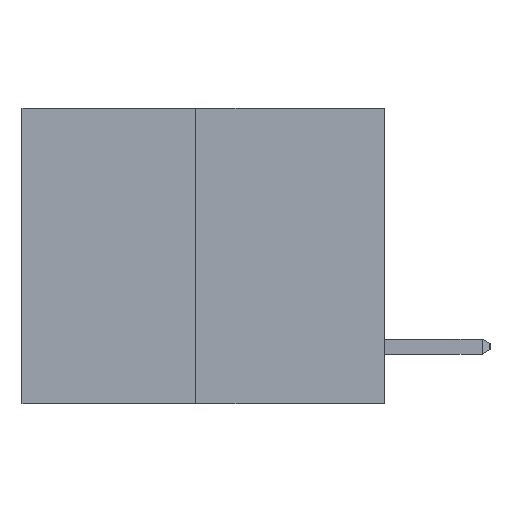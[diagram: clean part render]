
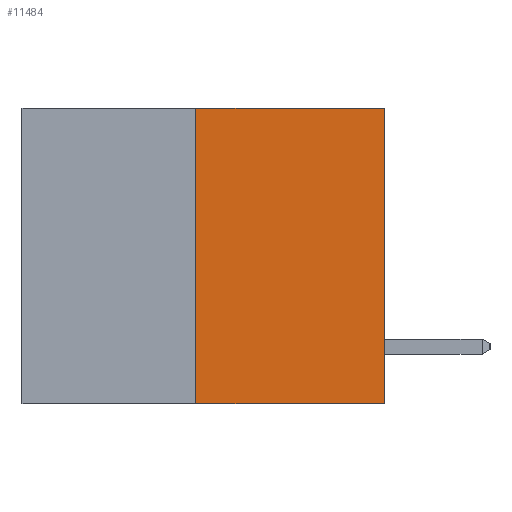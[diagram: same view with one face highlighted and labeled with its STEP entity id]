
A CAD part, left-side view. The second image highlights one B-rep face of the part: STEP entity #11484.
In plain terms, the highlighted planar face has unit normal (-1, 0, 0).
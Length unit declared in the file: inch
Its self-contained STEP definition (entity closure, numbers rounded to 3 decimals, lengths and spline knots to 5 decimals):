
#1360 = ORIENTED_EDGE ( 'NONE', *, *, #4857, .T. ) ;
#1458 = DIRECTION ( 'NONE',  ( 0., 0., 1. ) ) ;
#2323 = ORIENTED_EDGE ( 'NONE', *, *, #9073, .T. ) ;
#2783 = CARTESIAN_POINT ( 'NONE',  ( 0., 0.312, -0.49 ) ) ;
#3047 = VERTEX_POINT ( 'NONE', #7155 ) ;
#3718 = DIRECTION ( 'NONE',  ( 1., 0., 0. ) ) ;
#4088 = CARTESIAN_POINT ( 'NONE',  ( 0., 0., 0. ) ) ;
#4324 = CARTESIAN_POINT ( 'NONE',  ( 0., 0.312, 0. ) ) ;
#4562 = ORIENTED_EDGE ( 'NONE', *, *, #13847, .F. ) ;
#4671 = LINE ( 'NONE', #8353, #8855 ) ;
#4857 = EDGE_CURVE ( 'NONE', #11844, #3047, #4671, .T. ) ;
#4933 = DIRECTION ( 'NONE',  ( 0., 0., -1. ) ) ;
#5059 = CARTESIAN_POINT ( 'NONE',  ( 0., 0., 0. ) ) ;
#5150 = FACE_OUTER_BOUND ( 'NONE', #14146, .T. ) ;
#6136 = CARTESIAN_POINT ( 'NONE',  ( 0., 0.6, 0. ) ) ;
#6342 = DIRECTION ( 'NONE',  ( 0., 0., 1. ) ) ;
#7155 = CARTESIAN_POINT ( 'NONE',  ( 0., 0., -0.49 ) ) ;
#7371 = LINE ( 'NONE', #2783, #8485 ) ;
#8047 = CARTESIAN_POINT ( 'NONE',  ( 0., 0.312, -0.49 ) ) ;
#8353 = CARTESIAN_POINT ( 'NONE',  ( 0., 0.6, -0.49 ) ) ;
#8485 = VECTOR ( 'NONE', #1458, 39.37008 ) ;
#8506 = PLANE ( 'NONE',  #12933 ) ;
#8855 = VECTOR ( 'NONE', #9572, 39.37008 ) ;
#8947 = ORIENTED_EDGE ( 'NONE', *, *, #14756, .F. ) ;
#9073 = EDGE_CURVE ( 'NONE', #3047, #12836, #12267, .T. ) ;
#9205 = VECTOR ( 'NONE', #6342, 39.37008 ) ;
#9572 = DIRECTION ( 'NONE',  ( 0., -1., 0. ) ) ;
#10621 = DIRECTION ( 'NONE',  ( 0., -1., 0. ) ) ;
#11484 = ADVANCED_FACE ( 'NONE', ( #5150 ), #8506, .F. ) ;
#11517 = LINE ( 'NONE', #11868, #14362 ) ;
#11844 = VERTEX_POINT ( 'NONE', #8047 ) ;
#11868 = CARTESIAN_POINT ( 'NONE',  ( 0., 0.6, 0. ) ) ;
#12267 = LINE ( 'NONE', #4088, #9205 ) ;
#12836 = VERTEX_POINT ( 'NONE', #5059 ) ;
#12933 = AXIS2_PLACEMENT_3D ( 'NONE', #6136, #3718, #4933 ) ;
#13057 = VERTEX_POINT ( 'NONE', #4324 ) ;
#13847 = EDGE_CURVE ( 'NONE', #11844, #13057, #7371, .T. ) ;
#14146 = EDGE_LOOP ( 'NONE', ( #4562, #1360, #2323, #8947 ) ) ;
#14362 = VECTOR ( 'NONE', #10621, 39.37008 ) ;
#14756 = EDGE_CURVE ( 'NONE', #13057, #12836, #11517, .T. ) ;
